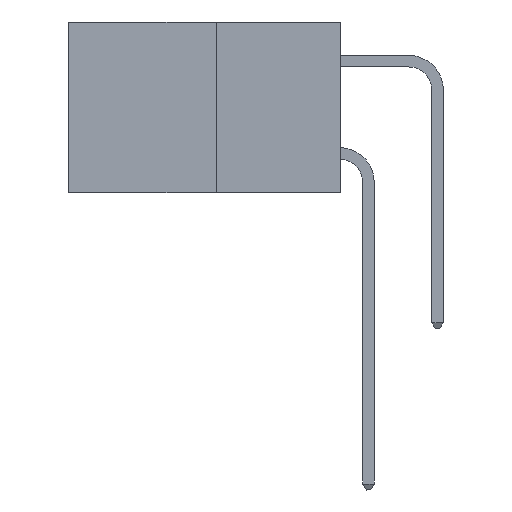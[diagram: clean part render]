
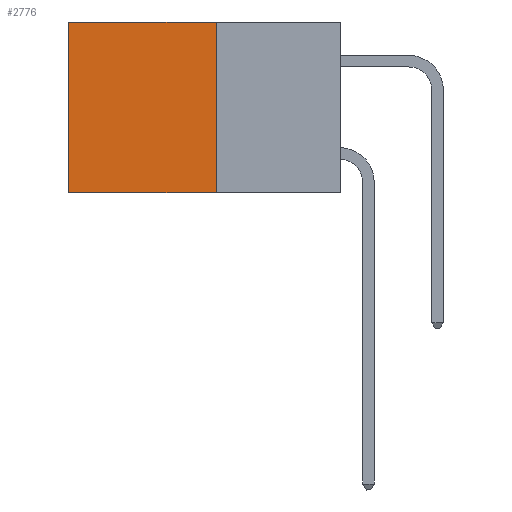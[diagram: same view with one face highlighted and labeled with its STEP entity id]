
A CAD part, left-side view. The second image highlights one B-rep face of the part: STEP entity #2776.
In plain terms, the highlighted planar face has unit normal (-1, 0, 0).
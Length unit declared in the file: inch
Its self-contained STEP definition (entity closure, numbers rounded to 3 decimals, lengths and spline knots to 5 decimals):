
#1171 = DIRECTION ( 'NONE',  ( 0., 1., 0. ) ) ;
#1402 = AXIS2_PLACEMENT_3D ( 'NONE', #3870, #10190, #24596 ) ;
#2014 = VERTEX_POINT ( 'NONE', #5370 ) ;
#2360 = ORIENTED_EDGE ( 'NONE', *, *, #19249, .T. ) ;
#2776 = ADVANCED_FACE ( 'NONE', ( #5552 ), #8080, .F. ) ;
#2788 = CARTESIAN_POINT ( 'NONE',  ( 0.277, 0.59, -0.37 ) ) ;
#3566 = VERTEX_POINT ( 'NONE', #12421 ) ;
#3870 = CARTESIAN_POINT ( 'NONE',  ( 0.277, 0.27, -0.37 ) ) ;
#4823 = EDGE_CURVE ( 'NONE', #10654, #2014, #14681, .T. ) ;
#4824 = ORIENTED_EDGE ( 'NONE', *, *, #24616, .T. ) ;
#5039 = LINE ( 'NONE', #17541, #15453 ) ;
#5370 = CARTESIAN_POINT ( 'NONE',  ( 0.277, 0.59, -0.37 ) ) ;
#5552 = FACE_OUTER_BOUND ( 'NONE', #25794, .T. ) ;
#8080 = PLANE ( 'NONE',  #1402 ) ;
#8262 = DIRECTION ( 'NONE',  ( 0., 1., 0. ) ) ;
#9755 = VERTEX_POINT ( 'NONE', #25803 ) ;
#10190 = DIRECTION ( 'NONE',  ( 1., 0., 0. ) ) ;
#10370 = CARTESIAN_POINT ( 'NONE',  ( 0.277, 0.27, -0.37 ) ) ;
#10654 = VERTEX_POINT ( 'NONE', #18551 ) ;
#12421 = CARTESIAN_POINT ( 'NONE',  ( 0.277, 0.59, 0. ) ) ;
#13283 = VECTOR ( 'NONE', #17289, 39.37008 ) ;
#14023 = VECTOR ( 'NONE', #8262, 39.37008 ) ;
#14661 = VECTOR ( 'NONE', #1171, 39.37008 ) ;
#14681 = LINE ( 'NONE', #10370, #14023 ) ;
#14683 = ORIENTED_EDGE ( 'NONE', *, *, #4823, .F. ) ;
#15453 = VECTOR ( 'NONE', #21698, 39.37008 ) ;
#17289 = DIRECTION ( 'NONE',  ( 0., 0., -1. ) ) ;
#17541 = CARTESIAN_POINT ( 'NONE',  ( 0.277, 0.27, -0.37 ) ) ;
#17762 = ORIENTED_EDGE ( 'NONE', *, *, #22139, .F. ) ;
#18551 = CARTESIAN_POINT ( 'NONE',  ( 0.277, 0.27, -0.37 ) ) ;
#19249 = EDGE_CURVE ( 'NONE', #9755, #3566, #20111, .T. ) ;
#20111 = LINE ( 'NONE', #25986, #14661 ) ;
#21698 = DIRECTION ( 'NONE',  ( 0., 0., -1. ) ) ;
#22139 = EDGE_CURVE ( 'NONE', #9755, #10654, #5039, .T. ) ;
#22952 = LINE ( 'NONE', #2788, #13283 ) ;
#24596 = DIRECTION ( 'NONE',  ( 0., 0., -1. ) ) ;
#24616 = EDGE_CURVE ( 'NONE', #3566, #2014, #22952, .T. ) ;
#25794 = EDGE_LOOP ( 'NONE', ( #4824, #14683, #17762, #2360 ) ) ;
#25803 = CARTESIAN_POINT ( 'NONE',  ( 0.277, 0.27, 0. ) ) ;
#25986 = CARTESIAN_POINT ( 'NONE',  ( 0.277, 0.27, 0. ) ) ;
